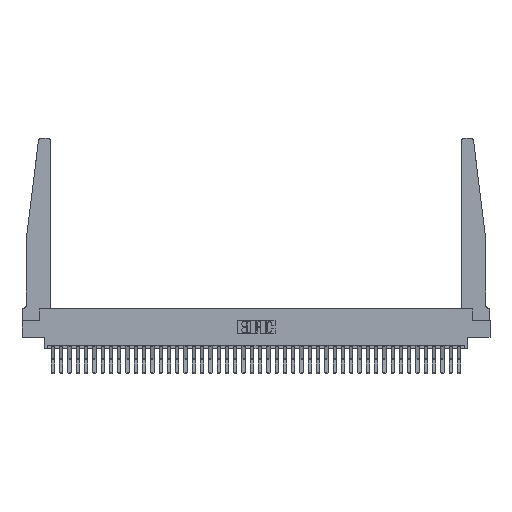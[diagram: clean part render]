
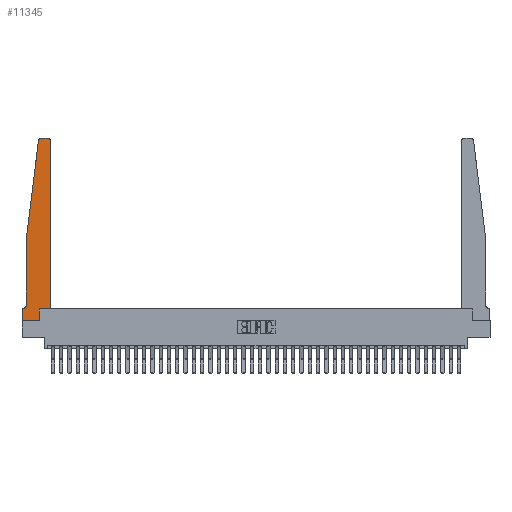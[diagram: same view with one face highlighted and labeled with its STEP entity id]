
A CAD part, top view. The second image highlights one B-rep face of the part: STEP entity #11345.
In plain terms, the highlighted planar face has unit normal (0, 0, 1).
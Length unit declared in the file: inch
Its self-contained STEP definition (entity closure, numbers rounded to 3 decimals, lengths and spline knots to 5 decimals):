
#505 = ORIENTED_EDGE ( 'NONE', *, *, #26074, .T. ) ;
#540 = FACE_OUTER_BOUND ( 'NONE', #9008, .T. ) ;
#874 = DIRECTION ( 'NONE',  ( -1., 0., 0. ) ) ;
#1331 = VERTEX_POINT ( 'NONE', #36499 ) ;
#2872 = EDGE_CURVE ( 'NONE', #34110, #1331, #8667, .T. ) ;
#2912 = CARTESIAN_POINT ( 'NONE',  ( 0.065, 1.25, 0.37 ) ) ;
#3223 = CIRCLE ( 'NONE', #10984, 0.03 ) ;
#3679 = CARTESIAN_POINT ( 'NONE',  ( 0.24675, 2.72367, 0.37 ) ) ;
#3904 = DIRECTION ( 'NONE',  ( 0., 0., 1. ) ) ;
#4107 = EDGE_CURVE ( 'NONE', #19653, #5715, #9923, .T. ) ;
#4280 = DIRECTION ( 'NONE',  ( 0., 0., -1. ) ) ;
#4459 = VECTOR ( 'NONE', #874, 39.37008 ) ;
#5545 = CARTESIAN_POINT ( 'NONE',  ( 0., 0.1875, 0.37 ) ) ;
#5637 = EDGE_CURVE ( 'NONE', #1331, #25482, #29345, .T. ) ;
#5715 = VERTEX_POINT ( 'NONE', #3679 ) ;
#6432 = CARTESIAN_POINT ( 'NONE',  ( 0., 0., 0.37 ) ) ;
#6724 = LINE ( 'NONE', #9531, #23306 ) ;
#6768 = CARTESIAN_POINT ( 'NONE',  ( 0., 0., 0.37 ) ) ;
#7396 = ORIENTED_EDGE ( 'NONE', *, *, #27505, .T. ) ;
#7816 = ORIENTED_EDGE ( 'NONE', *, *, #2872, .T. ) ;
#8514 = VECTOR ( 'NONE', #18099, 39.37008 ) ;
#8667 = CIRCLE ( 'NONE', #34971, 0.05 ) ;
#8748 = CARTESIAN_POINT ( 'NONE',  ( 0.065, 0.1875, 0.37 ) ) ;
#9001 = ORIENTED_EDGE ( 'NONE', *, *, #9873, .T. ) ;
#9008 = EDGE_LOOP ( 'NONE', ( #9001, #35009, #24508, #33503, #7816, #15480, #31233, #14272, #7396, #17008, #505, #18543 ) ) ;
#9281 = LINE ( 'NONE', #34556, #14450 ) ;
#9531 = CARTESIAN_POINT ( 'NONE',  ( 0.425, 0.18, 0.37 ) ) ;
#9873 = EDGE_CURVE ( 'NONE', #14788, #19653, #15275, .T. ) ;
#9923 = CIRCLE ( 'NONE', #30864, 0.03 ) ;
#10017 = CARTESIAN_POINT ( 'NONE',  ( 0.25, 2.75, 0.37 ) ) ;
#10984 = AXIS2_PLACEMENT_3D ( 'NONE', #30830, #24651, #15851 ) ;
#11345 = ADVANCED_FACE ( 'NONE', ( #540 ), #20940, .T. ) ;
#11740 = VECTOR ( 'NONE', #17853, 39.37008 ) ;
#11814 = VECTOR ( 'NONE', #30638, 39.37008 ) ;
#12074 = CARTESIAN_POINT ( 'NONE',  ( 0.065, 1.25, 0.37 ) ) ;
#12532 = CARTESIAN_POINT ( 'NONE',  ( 0.015, 0.2375, 0.37 ) ) ;
#12620 = VECTOR ( 'NONE', #29503, 39.37008 ) ;
#12948 = CARTESIAN_POINT ( 'NONE',  ( 0.425, 0.18, 0.37 ) ) ;
#14272 = ORIENTED_EDGE ( 'NONE', *, *, #29552, .T. ) ;
#14450 = VECTOR ( 'NONE', #29514, 39.37008 ) ;
#14788 = VERTEX_POINT ( 'NONE', #26185 ) ;
#15275 = LINE ( 'NONE', #10017, #4459 ) ;
#15480 = ORIENTED_EDGE ( 'NONE', *, *, #5637, .T. ) ;
#15851 = DIRECTION ( 'NONE',  ( 1., 0., 0. ) ) ;
#16125 = CARTESIAN_POINT ( 'NONE',  ( 0.27653, 2.75, 0.37 ) ) ;
#17008 = ORIENTED_EDGE ( 'NONE', *, *, #23002, .T. ) ;
#17393 = DIRECTION ( 'NONE',  ( 1., 0., 0. ) ) ;
#17465 = DIRECTION ( 'NONE',  ( 0., 1., 0. ) ) ;
#17688 = VERTEX_POINT ( 'NONE', #32753 ) ;
#17772 = CARTESIAN_POINT ( 'NONE',  ( 0., 0.1875, 0.37 ) ) ;
#17853 = DIRECTION ( 'NONE',  ( 0., -1., 0. ) ) ;
#18067 = LINE ( 'NONE', #12074, #12620 ) ;
#18099 = DIRECTION ( 'NONE',  ( -1., 0., 0. ) ) ;
#18543 = ORIENTED_EDGE ( 'NONE', *, *, #33528, .T. ) ;
#19034 = LINE ( 'NONE', #30456, #11814 ) ;
#19195 = CARTESIAN_POINT ( 'NONE',  ( 0.065, 1.25, 0.37 ) ) ;
#19448 = EDGE_CURVE ( 'NONE', #25482, #25668, #32094, .T. ) ;
#19653 = VERTEX_POINT ( 'NONE', #16125 ) ;
#20276 = LINE ( 'NONE', #26937, #31720 ) ;
#20737 = VERTEX_POINT ( 'NONE', #34525 ) ;
#20940 = PLANE ( 'NONE',  #22169 ) ;
#22169 = AXIS2_PLACEMENT_3D ( 'NONE', #17772, #3904, #17393 ) ;
#23002 = EDGE_CURVE ( 'NONE', #31055, #31239, #19034, .T. ) ;
#23222 = DIRECTION ( 'NONE',  ( 0., 1., 0. ) ) ;
#23306 = VECTOR ( 'NONE', #23222, 39.37008 ) ;
#24508 = ORIENTED_EDGE ( 'NONE', *, *, #28368, .T. ) ;
#24651 = DIRECTION ( 'NONE',  ( 0., 0., 1. ) ) ;
#24995 = DIRECTION ( 'NONE',  ( 0., -1., 0. ) ) ;
#25482 = VERTEX_POINT ( 'NONE', #5545 ) ;
#25668 = VERTEX_POINT ( 'NONE', #6768 ) ;
#26074 = EDGE_CURVE ( 'NONE', #31239, #17688, #6724, .T. ) ;
#26161 = CARTESIAN_POINT ( 'NONE',  ( 0.065, 0.2375, 0.37 ) ) ;
#26185 = CARTESIAN_POINT ( 'NONE',  ( 0.395, 2.75, 0.37 ) ) ;
#26937 = CARTESIAN_POINT ( 'NONE',  ( 0.2605, 0.18, 0.37 ) ) ;
#26939 = DIRECTION ( 'NONE',  ( -1., 0., 0. ) ) ;
#27505 = EDGE_CURVE ( 'NONE', #20737, #31055, #20276, .T. ) ;
#28368 = EDGE_CURVE ( 'NONE', #5715, #32481, #18067, .T. ) ;
#29345 = LINE ( 'NONE', #8748, #8514 ) ;
#29503 = DIRECTION ( 'NONE',  ( -0.122, -0.992, 0. ) ) ;
#29514 = DIRECTION ( 'NONE',  ( 1., 0., 0. ) ) ;
#29552 = EDGE_CURVE ( 'NONE', #25668, #20737, #9281, .T. ) ;
#30456 = CARTESIAN_POINT ( 'NONE',  ( 0.425, 0.18, 0.37 ) ) ;
#30638 = DIRECTION ( 'NONE',  ( 1., 0., 0. ) ) ;
#30826 = VECTOR ( 'NONE', #24995, 39.37008 ) ;
#30830 = CARTESIAN_POINT ( 'NONE',  ( 0.395, 2.72, 0.37 ) ) ;
#30864 = AXIS2_PLACEMENT_3D ( 'NONE', #31135, #31704, #34691 ) ;
#31055 = VERTEX_POINT ( 'NONE', #31172 ) ;
#31135 = CARTESIAN_POINT ( 'NONE',  ( 0.27653, 2.72, 0.37 ) ) ;
#31172 = CARTESIAN_POINT ( 'NONE',  ( 0.2605, 0.18, 0.37 ) ) ;
#31233 = ORIENTED_EDGE ( 'NONE', *, *, #19448, .T. ) ;
#31239 = VERTEX_POINT ( 'NONE', #12948 ) ;
#31704 = DIRECTION ( 'NONE',  ( 0., 0., 1. ) ) ;
#31720 = VECTOR ( 'NONE', #17465, 39.37008 ) ;
#32094 = LINE ( 'NONE', #6432, #11740 ) ;
#32481 = VERTEX_POINT ( 'NONE', #2912 ) ;
#32753 = CARTESIAN_POINT ( 'NONE',  ( 0.425, 2.72, 0.37 ) ) ;
#33439 = LINE ( 'NONE', #19195, #30826 ) ;
#33503 = ORIENTED_EDGE ( 'NONE', *, *, #35849, .T. ) ;
#33528 = EDGE_CURVE ( 'NONE', #17688, #14788, #3223, .T. ) ;
#34110 = VERTEX_POINT ( 'NONE', #26161 ) ;
#34525 = CARTESIAN_POINT ( 'NONE',  ( 0.2605, 0., 0.37 ) ) ;
#34556 = CARTESIAN_POINT ( 'NONE',  ( 0., 0., 0.37 ) ) ;
#34691 = DIRECTION ( 'NONE',  ( 1., 0., 0. ) ) ;
#34971 = AXIS2_PLACEMENT_3D ( 'NONE', #12532, #4280, #26939 ) ;
#35009 = ORIENTED_EDGE ( 'NONE', *, *, #4107, .T. ) ;
#35849 = EDGE_CURVE ( 'NONE', #32481, #34110, #33439, .T. ) ;
#36499 = CARTESIAN_POINT ( 'NONE',  ( 0.015, 0.1875, 0.37 ) ) ;
